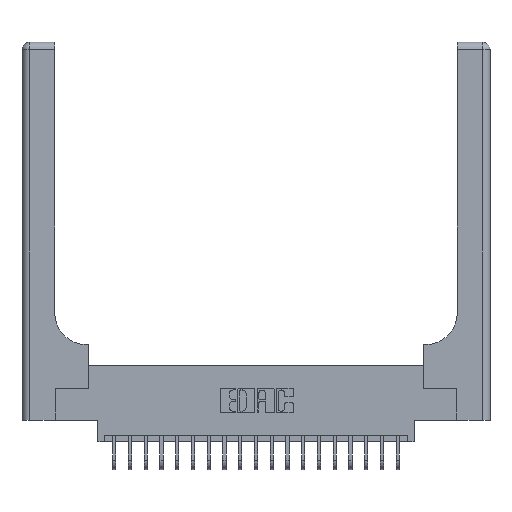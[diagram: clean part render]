
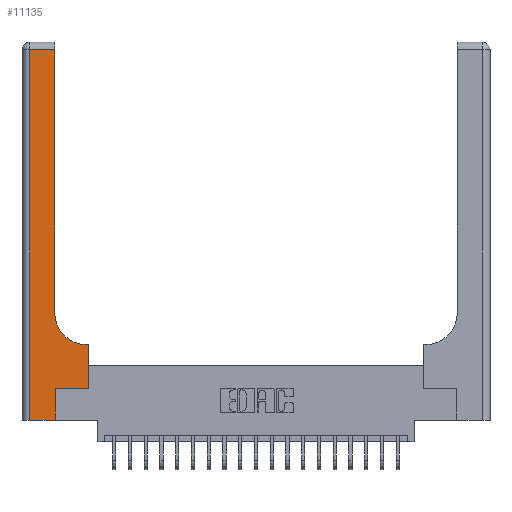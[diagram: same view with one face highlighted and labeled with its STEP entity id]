
A CAD part, top view. The second image highlights one B-rep face of the part: STEP entity #11135.
In plain terms, the highlighted planar face has unit normal (0, 0, 1).
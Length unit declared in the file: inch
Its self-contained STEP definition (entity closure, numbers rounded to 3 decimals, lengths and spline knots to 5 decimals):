
#505 = ORIENTED_EDGE ( 'NONE', *, *, #14145, .T. ) ;
#933 = VERTEX_POINT ( 'NONE', #17955 ) ;
#999 = DIRECTION ( 'NONE',  ( 0., 0., -1. ) ) ;
#1073 = ORIENTED_EDGE ( 'NONE', *, *, #16714, .T. ) ;
#1615 = VERTEX_POINT ( 'NONE', #8131 ) ;
#1902 = CARTESIAN_POINT ( 'NONE',  ( 0.26, 0.6, 0.37 ) ) ;
#2130 = CARTESIAN_POINT ( 'NONE',  ( 0.06, 3., 0.37 ) ) ;
#2308 = CARTESIAN_POINT ( 'NONE',  ( 0., 0., 0.37 ) ) ;
#2804 = CARTESIAN_POINT ( 'NONE',  ( 0.528, 0.25, 0.37 ) ) ;
#3197 = VECTOR ( 'NONE', #11819, 39.37008 ) ;
#3259 = ORIENTED_EDGE ( 'NONE', *, *, #18218, .T. ) ;
#3378 = FACE_OUTER_BOUND ( 'NONE', #22577, .T. ) ;
#3869 = VECTOR ( 'NONE', #11796, 39.37008 ) ;
#4029 = LINE ( 'NONE', #11036, #7846 ) ;
#4449 = VERTEX_POINT ( 'NONE', #20629 ) ;
#4544 = DIRECTION ( 'NONE',  ( 0., 1., 0. ) ) ;
#4613 = AXIS2_PLACEMENT_3D ( 'NONE', #21554, #19582, #15969 ) ;
#5061 = EDGE_CURVE ( 'NONE', #1615, #7354, #4029, .T. ) ;
#5566 = DIRECTION ( 'NONE',  ( 1., 0., 0. ) ) ;
#5795 = ORIENTED_EDGE ( 'NONE', *, *, #20442, .T. ) ;
#6177 = ORIENTED_EDGE ( 'NONE', *, *, #5061, .T. ) ;
#6258 = CARTESIAN_POINT ( 'NONE',  ( 0.26, 2.94, 0.37 ) ) ;
#6300 = CARTESIAN_POINT ( 'NONE',  ( 0.265, 0., 0.37 ) ) ;
#6882 = CARTESIAN_POINT ( 'NONE',  ( 0.265, 0., 0.37 ) ) ;
#7015 = ORIENTED_EDGE ( 'NONE', *, *, #16766, .T. ) ;
#7129 = LINE ( 'NONE', #14345, #15368 ) ;
#7295 = CIRCLE ( 'NONE', #10264, 0.25 ) ;
#7354 = VERTEX_POINT ( 'NONE', #18752 ) ;
#7807 = DIRECTION ( 'NONE',  ( 1., 0., 0. ) ) ;
#7812 = VERTEX_POINT ( 'NONE', #6258 ) ;
#7844 = ORIENTED_EDGE ( 'NONE', *, *, #13174, .T. ) ;
#7846 = VECTOR ( 'NONE', #5566, 39.37008 ) ;
#8131 = CARTESIAN_POINT ( 'NONE',  ( 0.265, 0.25, 0.37 ) ) ;
#8359 = VECTOR ( 'NONE', #7807, 39.37008 ) ;
#8678 = VECTOR ( 'NONE', #4544, 39.37008 ) ;
#9734 = CARTESIAN_POINT ( 'NONE',  ( 0.26, 3., 0.37 ) ) ;
#10160 = ORIENTED_EDGE ( 'NONE', *, *, #17473, .T. ) ;
#10264 = AXIS2_PLACEMENT_3D ( 'NONE', #18730, #999, #20697 ) ;
#10404 = CARTESIAN_POINT ( 'NONE',  ( 0.06, 2.94, 0.37 ) ) ;
#10836 = CARTESIAN_POINT ( 'NONE',  ( 0.528, 0.6, 0.37 ) ) ;
#10963 = PLANE ( 'NONE',  #4613 ) ;
#11036 = CARTESIAN_POINT ( 'NONE',  ( 0.265, 0.25, 0.37 ) ) ;
#11135 = ADVANCED_FACE ( 'NONE', ( #3378 ), #10963, .F. ) ;
#11405 = ORIENTED_EDGE ( 'NONE', *, *, #19963, .T. ) ;
#11796 = DIRECTION ( 'NONE',  ( 0., 1., 0. ) ) ;
#11819 = DIRECTION ( 'NONE',  ( 0., 1., 0. ) ) ;
#12059 = DIRECTION ( 'NONE',  ( -1., 0., 0. ) ) ;
#13174 = EDGE_CURVE ( 'NONE', #7354, #15146, #21950, .T. ) ;
#14145 = EDGE_CURVE ( 'NONE', #15146, #4449, #22898, .T. ) ;
#14224 = DIRECTION ( 'NONE',  ( -1., 0., 0. ) ) ;
#14345 = CARTESIAN_POINT ( 'NONE',  ( 0., 2.94, 0.37 ) ) ;
#14606 = LINE ( 'NONE', #2130, #21726 ) ;
#15146 = VERTEX_POINT ( 'NONE', #10836 ) ;
#15314 = LINE ( 'NONE', #9734, #3197 ) ;
#15368 = VECTOR ( 'NONE', #14224, 39.37008 ) ;
#15882 = VERTEX_POINT ( 'NONE', #10404 ) ;
#15969 = DIRECTION ( 'NONE',  ( -1., 0., 0. ) ) ;
#16714 = EDGE_CURVE ( 'NONE', #7812, #15882, #7129, .T. ) ;
#16766 = EDGE_CURVE ( 'NONE', #19225, #1615, #22039, .T. ) ;
#16769 = LINE ( 'NONE', #2308, #8359 ) ;
#17092 = VERTEX_POINT ( 'NONE', #21743 ) ;
#17473 = EDGE_CURVE ( 'NONE', #15882, #17092, #14606, .T. ) ;
#17955 = CARTESIAN_POINT ( 'NONE',  ( 0.26, 0.85, 0.37 ) ) ;
#18218 = EDGE_CURVE ( 'NONE', #17092, #19225, #16769, .T. ) ;
#18730 = CARTESIAN_POINT ( 'NONE',  ( 0.51, 0.85, 0.37 ) ) ;
#18752 = CARTESIAN_POINT ( 'NONE',  ( 0.528, 0.25, 0.37 ) ) ;
#19225 = VERTEX_POINT ( 'NONE', #6882 ) ;
#19582 = DIRECTION ( 'NONE',  ( 0., 0., -1. ) ) ;
#19963 = EDGE_CURVE ( 'NONE', #4449, #933, #7295, .T. ) ;
#19971 = DIRECTION ( 'NONE',  ( 0., -1., 0. ) ) ;
#20442 = EDGE_CURVE ( 'NONE', #933, #7812, #15314, .T. ) ;
#20629 = CARTESIAN_POINT ( 'NONE',  ( 0.51, 0.6, 0.37 ) ) ;
#20697 = DIRECTION ( 'NONE',  ( 1., 0., 0. ) ) ;
#21386 = VECTOR ( 'NONE', #12059, 39.37008 ) ;
#21554 = CARTESIAN_POINT ( 'NONE',  ( 0., 3., 0.37 ) ) ;
#21726 = VECTOR ( 'NONE', #19971, 39.37008 ) ;
#21743 = CARTESIAN_POINT ( 'NONE',  ( 0.06, 0., 0.37 ) ) ;
#21950 = LINE ( 'NONE', #2804, #3869 ) ;
#22039 = LINE ( 'NONE', #6300, #8678 ) ;
#22577 = EDGE_LOOP ( 'NONE', ( #5795, #1073, #10160, #3259, #7015, #6177, #7844, #505, #11405 ) ) ;
#22898 = LINE ( 'NONE', #1902, #21386 ) ;
